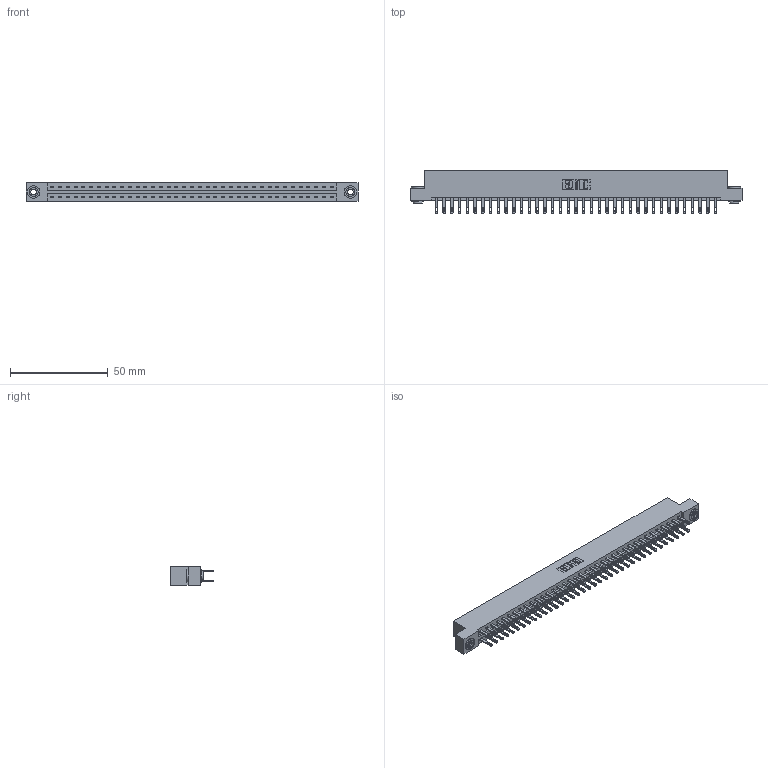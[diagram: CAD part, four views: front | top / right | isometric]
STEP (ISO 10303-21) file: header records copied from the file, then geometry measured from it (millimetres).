
FILE_DESCRIPTION (( 'STEP AP203' ), '1' );
FILE_NAME ('887-074-500-203.STEP', '2020-09-21T03:36:57', ( '' ), ( '' ), 'SwSTEP 2.0', 'SolidWorks 2020', '' );
FILE_SCHEMA (( 'CONFIG_CONTROL_DESIGN' ));
Length unit declared in the file: inch
Products named in the file (4): 837 Part_Flush Mounting Lugs - 0.156 Dia-TH; 345-250-002_345-250-002-102; 345-292-001_345-293-100; 887-074-500-203
Assembly tree (77 placements, depth 2):
  887-074-500-203
    837 Part_Flush Mounting Lugs - 0.156 Dia-TH
    345-292-001_345-293-100  x74
    345-250-002_345-250-002-102  x2
Bounding box: 169.62 x 21.85 x 9.4 mm (x, y, z)
Volume: 18055 mm3; surface area: 21408.1 mm2
Topology: 77 solids, 77 shells, 3852 faces, 11709 edges, 7802 vertices
Faces by surface type: plane 2448, cylinder 1396, cone 8
Entity records: 29914 total; most frequent: CARTESIAN_POINT 5017, ORIENTED_EDGE 4946, DIRECTION 4311, EDGE_CURVE 2473, VECTOR 2317, LINE 2317, VERTEX_POINT 1646, AXIS2_PLACEMENT_3D 997
